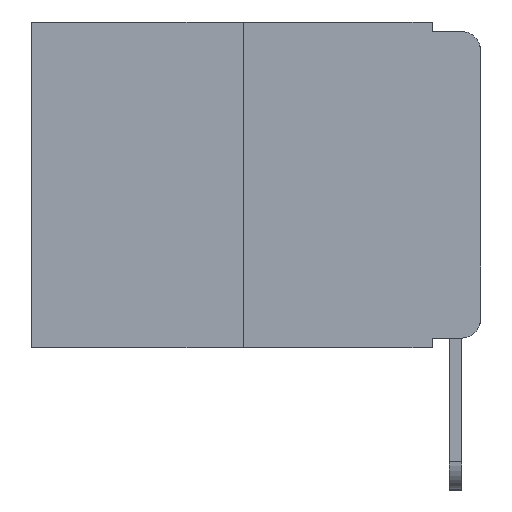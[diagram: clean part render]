
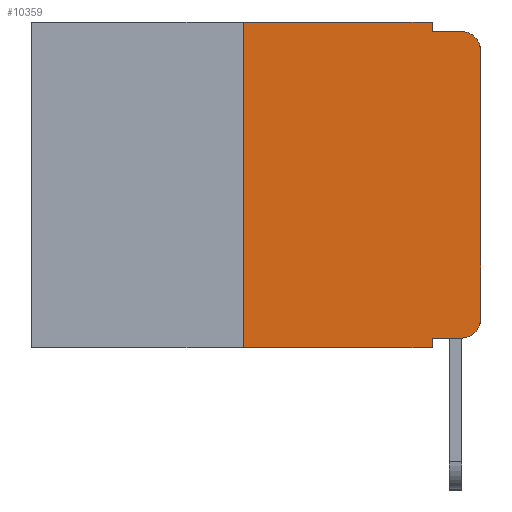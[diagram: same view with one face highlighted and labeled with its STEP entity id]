
A CAD part, left-side view. The second image highlights one B-rep face of the part: STEP entity #10359.
In plain terms, the highlighted planar face has unit normal (-1, 0, 0).
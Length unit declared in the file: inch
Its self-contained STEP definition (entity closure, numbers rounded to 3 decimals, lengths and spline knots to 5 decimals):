
#167 = LINE ( 'NONE', #2157, #11501 ) ;
#299 = AXIS2_PLACEMENT_3D ( 'NONE', #842, #11672, #10732 ) ;
#842 = CARTESIAN_POINT ( 'NONE',  ( 0., 0.02, -0.03 ) ) ;
#1042 = VERTEX_POINT ( 'NONE', #10497 ) ;
#1068 = VERTEX_POINT ( 'NONE', #8705 ) ;
#1310 = EDGE_LOOP ( 'NONE', ( #3540, #3479, #2766, #1784, #1601, #7516, #11411, #1904, #7117, #2401 ) ) ;
#1330 = DIRECTION ( 'NONE',  ( 0., 0., 1. ) ) ;
#1426 = VERTEX_POINT ( 'NONE', #6642 ) ;
#1464 = DIRECTION ( 'NONE',  ( 0., 0., -1. ) ) ;
#1601 = ORIENTED_EDGE ( 'NONE', *, *, #2470, .F. ) ;
#1638 = LINE ( 'NONE', #10688, #8375 ) ;
#1784 = ORIENTED_EDGE ( 'NONE', *, *, #1938, .F. ) ;
#1822 = EDGE_CURVE ( 'NONE', #7025, #1426, #167, .T. ) ;
#1855 = EDGE_CURVE ( 'NONE', #4942, #5700, #9102, .T. ) ;
#1904 = ORIENTED_EDGE ( 'NONE', *, *, #1855, .F. ) ;
#1938 = EDGE_CURVE ( 'NONE', #5190, #4570, #9582, .T. ) ;
#2137 = VERTEX_POINT ( 'NONE', #10697 ) ;
#2157 = CARTESIAN_POINT ( 'NONE',  ( 0., 0., 0. ) ) ;
#2177 = CARTESIAN_POINT ( 'NONE',  ( 0., 0.02, -0.313 ) ) ;
#2185 = CARTESIAN_POINT ( 'NONE',  ( 0., 0.051, -0.343 ) ) ;
#2401 = ORIENTED_EDGE ( 'NONE', *, *, #7467, .T. ) ;
#2470 = EDGE_CURVE ( 'NONE', #6219, #5190, #3423, .T. ) ;
#2540 = EDGE_CURVE ( 'NONE', #1068, #5700, #1638, .T. ) ;
#2602 = DIRECTION ( 'NONE',  ( 0., -1., 0. ) ) ;
#2766 = ORIENTED_EDGE ( 'NONE', *, *, #8792, .F. ) ;
#2976 = DIRECTION ( 'NONE',  ( 0., 0., -1. ) ) ;
#3061 = CARTESIAN_POINT ( 'NONE',  ( 0., 0., -0.313 ) ) ;
#3290 = CARTESIAN_POINT ( 'NONE',  ( 0., 0.051, -0.01 ) ) ;
#3372 = DIRECTION ( 'NONE',  ( 0., -1., 0. ) ) ;
#3423 = LINE ( 'NONE', #7192, #4395 ) ;
#3479 = ORIENTED_EDGE ( 'NONE', *, *, #4281, .T. ) ;
#3540 = ORIENTED_EDGE ( 'NONE', *, *, #1822, .T. ) ;
#3929 = DIRECTION ( 'NONE',  ( 0., 0., -1. ) ) ;
#4153 = AXIS2_PLACEMENT_3D ( 'NONE', #11071, #9280, #2976 ) ;
#4248 = CARTESIAN_POINT ( 'NONE',  ( 0., 0.051, -0.333 ) ) ;
#4281 = EDGE_CURVE ( 'NONE', #1426, #1042, #11090, .T. ) ;
#4395 = VECTOR ( 'NONE', #3372, 39.37008 ) ;
#4493 = VECTOR ( 'NONE', #6877, 39.37008 ) ;
#4570 = VERTEX_POINT ( 'NONE', #9477 ) ;
#4738 = AXIS2_PLACEMENT_3D ( 'NONE', #2177, #5705, #3929 ) ;
#4775 = CARTESIAN_POINT ( 'NONE',  ( 0., 0.25, 0. ) ) ;
#4942 = VERTEX_POINT ( 'NONE', #4248 ) ;
#5071 = VECTOR ( 'NONE', #1464, 39.37008 ) ;
#5190 = VERTEX_POINT ( 'NONE', #9144 ) ;
#5496 = CIRCLE ( 'NONE', #4738, 0.02 ) ;
#5685 = CARTESIAN_POINT ( 'NONE',  ( 0., 0.051, 0. ) ) ;
#5700 = VERTEX_POINT ( 'NONE', #2185 ) ;
#5705 = DIRECTION ( 'NONE',  ( -1., 0., 0. ) ) ;
#6219 = VERTEX_POINT ( 'NONE', #8793 ) ;
#6621 = EDGE_CURVE ( 'NONE', #1068, #6219, #9437, .T. ) ;
#6642 = CARTESIAN_POINT ( 'NONE',  ( 0., 0., -0.03 ) ) ;
#6652 = EDGE_CURVE ( 'NONE', #4942, #2137, #10274, .T. ) ;
#6844 = VECTOR ( 'NONE', #11422, 39.37008 ) ;
#6877 = DIRECTION ( 'NONE',  ( 0., 0., -1. ) ) ;
#6972 = CARTESIAN_POINT ( 'NONE',  ( 0., 0.051, -0.333 ) ) ;
#7025 = VERTEX_POINT ( 'NONE', #3061 ) ;
#7117 = ORIENTED_EDGE ( 'NONE', *, *, #6652, .T. ) ;
#7192 = CARTESIAN_POINT ( 'NONE',  ( 0., 0.473, 0. ) ) ;
#7467 = EDGE_CURVE ( 'NONE', #2137, #7025, #5496, .T. ) ;
#7516 = ORIENTED_EDGE ( 'NONE', *, *, #6621, .F. ) ;
#8375 = VECTOR ( 'NONE', #2602, 39.37008 ) ;
#8532 = VECTOR ( 'NONE', #10553, 39.37008 ) ;
#8705 = CARTESIAN_POINT ( 'NONE',  ( 0., 0.25, -0.343 ) ) ;
#8749 = CARTESIAN_POINT ( 'NONE',  ( 0., 0.051, 0. ) ) ;
#8792 = EDGE_CURVE ( 'NONE', #4570, #1042, #11450, .T. ) ;
#8793 = CARTESIAN_POINT ( 'NONE',  ( 0., 0.25, 0. ) ) ;
#8880 = VECTOR ( 'NONE', #1330, 39.37008 ) ;
#9102 = LINE ( 'NONE', #5685, #4493 ) ;
#9144 = CARTESIAN_POINT ( 'NONE',  ( 0., 0.051, 0. ) ) ;
#9162 = PLANE ( 'NONE',  #4153 ) ;
#9222 = FACE_OUTER_BOUND ( 'NONE', #1310, .T. ) ;
#9280 = DIRECTION ( 'NONE',  ( 1., 0., 0. ) ) ;
#9437 = LINE ( 'NONE', #4775, #8880 ) ;
#9477 = CARTESIAN_POINT ( 'NONE',  ( 0., 0.051, -0.01 ) ) ;
#9582 = LINE ( 'NONE', #8749, #5071 ) ;
#10168 = DIRECTION ( 'NONE',  ( 0., 0., 1. ) ) ;
#10274 = LINE ( 'NONE', #6972, #6844 ) ;
#10359 = ADVANCED_FACE ( 'NONE', ( #9222 ), #9162, .F. ) ;
#10497 = CARTESIAN_POINT ( 'NONE',  ( 0., 0.02, -0.01 ) ) ;
#10553 = DIRECTION ( 'NONE',  ( 0., -1., 0. ) ) ;
#10688 = CARTESIAN_POINT ( 'NONE',  ( 0., 0.473, -0.343 ) ) ;
#10697 = CARTESIAN_POINT ( 'NONE',  ( 0., 0.02, -0.333 ) ) ;
#10732 = DIRECTION ( 'NONE',  ( 0., 0., -1. ) ) ;
#11071 = CARTESIAN_POINT ( 'NONE',  ( 0., 0.473, 0. ) ) ;
#11090 = CIRCLE ( 'NONE', #299, 0.02 ) ;
#11411 = ORIENTED_EDGE ( 'NONE', *, *, #2540, .T. ) ;
#11422 = DIRECTION ( 'NONE',  ( 0., -1., 0. ) ) ;
#11450 = LINE ( 'NONE', #3290, #8532 ) ;
#11501 = VECTOR ( 'NONE', #10168, 39.37008 ) ;
#11672 = DIRECTION ( 'NONE',  ( -1., 0., 0. ) ) ;
